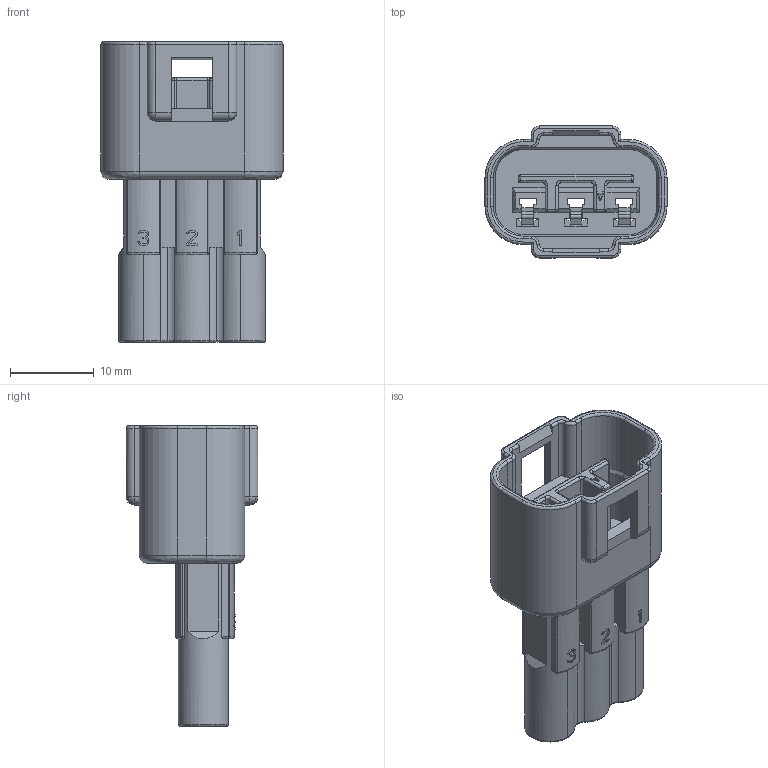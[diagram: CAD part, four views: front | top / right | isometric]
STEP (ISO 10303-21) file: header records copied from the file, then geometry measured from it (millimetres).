
FILE_DESCRIPTION (( 'STEP AP214' ), '1' );
FILE_NAME ('572-003-000-100.STEP', '2020-07-30T18:53:24', ( '' ), ( '' ), 'SwSTEP 2.0', 'SolidWorks 2020', '' );
FILE_SCHEMA (( 'AUTOMOTIVE_DESIGN' ));
Length unit declared in the file: millimetre
Products named in the file (1): 572-003-000-100
Bounding box: 21.8 x 15.8 x 36 mm (x, y, z)
Volume: 2516.5 mm3; surface area: 4768.5 mm2
Topology: 1 solids, 1 shells, 612 faces, 1655 edges, 1002 vertices
Faces by surface type: plane 349, cylinder 157, bspline 96, cone 10
Entity records: 20235 total; most frequent: CARTESIAN_POINT 5960, ORIENTED_EDGE 3222, DIRECTION 2750, EDGE_CURVE 1611, VERTEX_POINT 1002, LINE 944, VECTOR 944, AXIS2_PLACEMENT_3D 903
